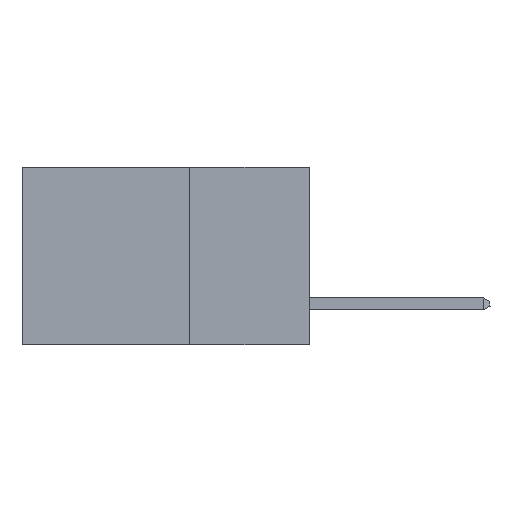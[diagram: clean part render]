
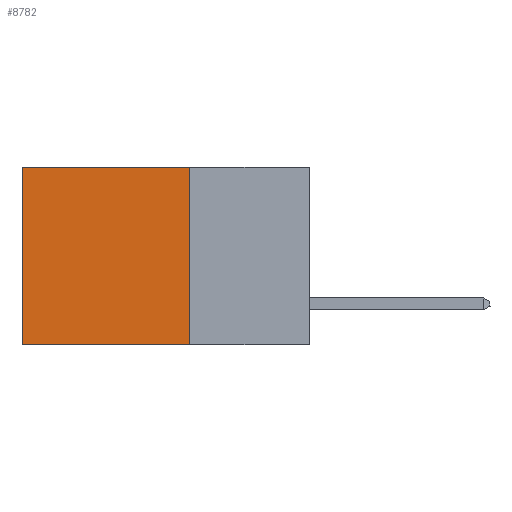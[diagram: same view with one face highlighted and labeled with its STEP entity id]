
A CAD part, left-side view. The second image highlights one B-rep face of the part: STEP entity #8782.
In plain terms, the highlighted planar face has unit normal (-1, 0, 0).
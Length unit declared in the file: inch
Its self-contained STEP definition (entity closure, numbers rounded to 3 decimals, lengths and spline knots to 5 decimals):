
#851 = EDGE_CURVE ( 'NONE', #12747, #3974, #3404, .T. ) ;
#2092 = EDGE_CURVE ( 'NONE', #26228, #3974, #28792, .T. ) ;
#2672 = EDGE_CURVE ( 'NONE', #31456, #26228, #27562, .T. ) ;
#3404 = LINE ( 'NONE', #6632, #13536 ) ;
#3974 = VERTEX_POINT ( 'NONE', #10686 ) ;
#4573 = EDGE_CURVE ( 'NONE', #31456, #12747, #10088, .T. ) ;
#6540 = DIRECTION ( 'NONE',  ( 0., 0., -1. ) ) ;
#6632 = CARTESIAN_POINT ( 'NONE',  ( 0.2875, 0.25, -0.37 ) ) ;
#8549 = VECTOR ( 'NONE', #29231, 39.37008 ) ;
#8782 = ADVANCED_FACE ( 'NONE', ( #32974 ), #12657, .F. ) ;
#9300 = CARTESIAN_POINT ( 'NONE',  ( 0.2875, 0.25, 0. ) ) ;
#9924 = DIRECTION ( 'NONE',  ( 0., 0., -1. ) ) ;
#10088 = LINE ( 'NONE', #11900, #16107 ) ;
#10686 = CARTESIAN_POINT ( 'NONE',  ( 0.2875, 0.6, -0.37 ) ) ;
#11336 = CARTESIAN_POINT ( 'NONE',  ( 0.2875, 0.6, 0. ) ) ;
#11900 = CARTESIAN_POINT ( 'NONE',  ( 0.2875, 0.25, 0. ) ) ;
#12657 = PLANE ( 'NONE',  #28967 ) ;
#12747 = VERTEX_POINT ( 'NONE', #17776 ) ;
#12865 = DIRECTION ( 'NONE',  ( 1., 0., 0. ) ) ;
#13397 = EDGE_LOOP ( 'NONE', ( #29305, #31339, #19132, #24688 ) ) ;
#13536 = VECTOR ( 'NONE', #13891, 39.37008 ) ;
#13792 = VECTOR ( 'NONE', #24827, 39.37008 ) ;
#13891 = DIRECTION ( 'NONE',  ( 0., 1., 0. ) ) ;
#16107 = VECTOR ( 'NONE', #6540, 39.37008 ) ;
#17776 = CARTESIAN_POINT ( 'NONE',  ( 0.2875, 0.25, -0.37 ) ) ;
#19132 = ORIENTED_EDGE ( 'NONE', *, *, #4573, .F. ) ;
#21310 = CARTESIAN_POINT ( 'NONE',  ( 0.2875, 0.6, 0. ) ) ;
#24688 = ORIENTED_EDGE ( 'NONE', *, *, #2672, .T. ) ;
#24827 = DIRECTION ( 'NONE',  ( 0., 1., 0. ) ) ;
#26228 = VERTEX_POINT ( 'NONE', #11336 ) ;
#27562 = LINE ( 'NONE', #30101, #13792 ) ;
#28792 = LINE ( 'NONE', #21310, #8549 ) ;
#28967 = AXIS2_PLACEMENT_3D ( 'NONE', #33292, #12865, #9924 ) ;
#29231 = DIRECTION ( 'NONE',  ( 0., 0., -1. ) ) ;
#29305 = ORIENTED_EDGE ( 'NONE', *, *, #2092, .T. ) ;
#30101 = CARTESIAN_POINT ( 'NONE',  ( 0.2875, 0.25, 0. ) ) ;
#31339 = ORIENTED_EDGE ( 'NONE', *, *, #851, .F. ) ;
#31456 = VERTEX_POINT ( 'NONE', #9300 ) ;
#32974 = FACE_OUTER_BOUND ( 'NONE', #13397, .T. ) ;
#33292 = CARTESIAN_POINT ( 'NONE',  ( 0.2875, 0.25, 0. ) ) ;
